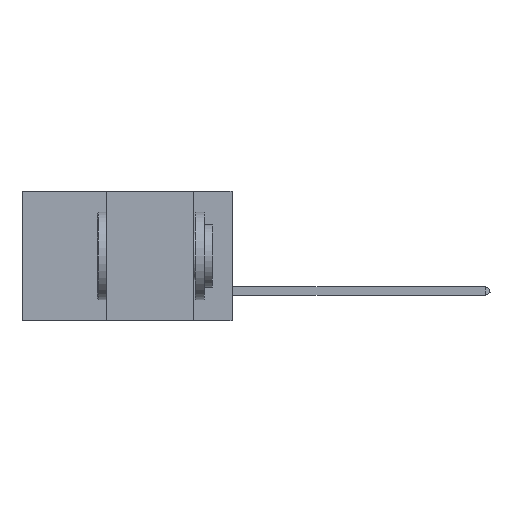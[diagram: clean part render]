
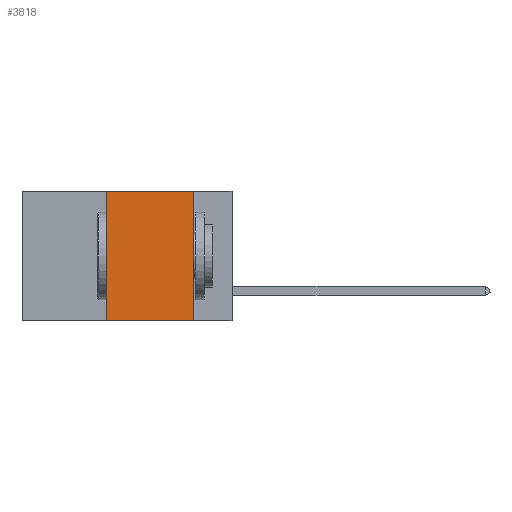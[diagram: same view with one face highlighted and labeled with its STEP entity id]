
A CAD part, left-side view. The second image highlights one B-rep face of the part: STEP entity #3818.
In plain terms, the highlighted planar face has unit normal (-1, 0, 0).
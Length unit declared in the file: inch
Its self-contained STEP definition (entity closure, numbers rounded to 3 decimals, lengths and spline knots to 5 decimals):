
#249 = CARTESIAN_POINT ( 'NONE',  ( 0., 0.11, -0.37 ) ) ;
#999 = ORIENTED_EDGE ( 'NONE', *, *, #7870, .F. ) ;
#1274 = PLANE ( 'NONE',  #5332 ) ;
#1382 = CARTESIAN_POINT ( 'NONE',  ( 0., 0.6, 0. ) ) ;
#1491 = EDGE_CURVE ( 'NONE', #6579, #2809, #10417, .T. ) ;
#1837 = ORIENTED_EDGE ( 'NONE', *, *, #4670, .F. ) ;
#2780 = CARTESIAN_POINT ( 'NONE',  ( 0., 0.36, 0. ) ) ;
#2809 = VERTEX_POINT ( 'NONE', #8385 ) ;
#3494 = VECTOR ( 'NONE', #10228, 39.37008 ) ;
#3682 = DIRECTION ( 'NONE',  ( 0., -1., 0. ) ) ;
#3818 = ADVANCED_FACE ( 'NONE', ( #4453 ), #1274, .F. ) ;
#3915 = CARTESIAN_POINT ( 'NONE',  ( 0., 0.36, 0. ) ) ;
#4295 = LINE ( 'NONE', #2780, #3494 ) ;
#4320 = DIRECTION ( 'NONE',  ( 0., -1., 0. ) ) ;
#4421 = VECTOR ( 'NONE', #9673, 39.37008 ) ;
#4453 = FACE_OUTER_BOUND ( 'NONE', #9378, .T. ) ;
#4670 = EDGE_CURVE ( 'NONE', #9132, #6579, #4295, .T. ) ;
#5145 = CARTESIAN_POINT ( 'NONE',  ( 0., 0.6, -0.37 ) ) ;
#5332 = AXIS2_PLACEMENT_3D ( 'NONE', #1382, #10450, #7236 ) ;
#5609 = CARTESIAN_POINT ( 'NONE',  ( 0., 0.36, -0.37 ) ) ;
#6383 = VERTEX_POINT ( 'NONE', #249 ) ;
#6579 = VERTEX_POINT ( 'NONE', #3915 ) ;
#7137 = ORIENTED_EDGE ( 'NONE', *, *, #1491, .F. ) ;
#7236 = DIRECTION ( 'NONE',  ( 0., 0., -1. ) ) ;
#7870 = EDGE_CURVE ( 'NONE', #2809, #6383, #10094, .T. ) ;
#8385 = CARTESIAN_POINT ( 'NONE',  ( 0., 0.11, 0. ) ) ;
#8762 = VECTOR ( 'NONE', #3682, 39.37008 ) ;
#8816 = EDGE_CURVE ( 'NONE', #9132, #6383, #9431, .T. ) ;
#8941 = CARTESIAN_POINT ( 'NONE',  ( 0., 0.11, 0. ) ) ;
#9132 = VERTEX_POINT ( 'NONE', #5609 ) ;
#9155 = ORIENTED_EDGE ( 'NONE', *, *, #8816, .T. ) ;
#9175 = VECTOR ( 'NONE', #4320, 39.37008 ) ;
#9378 = EDGE_LOOP ( 'NONE', ( #999, #7137, #1837, #9155 ) ) ;
#9431 = LINE ( 'NONE', #5145, #9175 ) ;
#9673 = DIRECTION ( 'NONE',  ( 0., 0., -1. ) ) ;
#10094 = LINE ( 'NONE', #8941, #4421 ) ;
#10228 = DIRECTION ( 'NONE',  ( 0., 0., 1. ) ) ;
#10362 = CARTESIAN_POINT ( 'NONE',  ( 0., 0.6, 0. ) ) ;
#10417 = LINE ( 'NONE', #10362, #8762 ) ;
#10450 = DIRECTION ( 'NONE',  ( 1., 0., 0. ) ) ;
